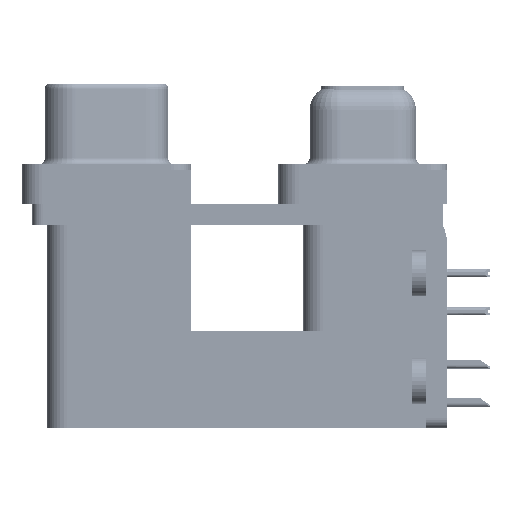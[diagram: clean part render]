
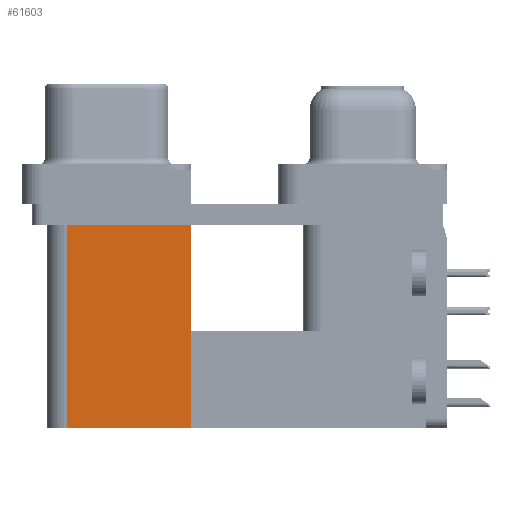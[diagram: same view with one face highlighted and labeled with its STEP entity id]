
A CAD part, left-side view. The second image highlights one B-rep face of the part: STEP entity #61603.
In plain terms, the highlighted planar face has unit normal (-1, 0, 0).
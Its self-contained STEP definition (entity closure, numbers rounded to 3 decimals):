
#1164 = VECTOR ( 'NONE', #51424, 1000. ) ;
#2717 = PLANE ( 'NONE',  #69820 ) ;
#3082 = CARTESIAN_POINT ( 'NONE',  ( 3.79, 12.775, -19.2 ) ) ;
#3786 = DIRECTION ( 'NONE',  ( 0., 1., 0. ) ) ;
#4133 = CARTESIAN_POINT ( 'NONE',  ( 3.79, 21.975, -19.2 ) ) ;
#6581 = ORIENTED_EDGE ( 'NONE', *, *, #23074, .F. ) ;
#8945 = CARTESIAN_POINT ( 'NONE',  ( 3.79, 12.775, -19.2 ) ) ;
#14215 = VECTOR ( 'NONE', #20012, 1000. ) ;
#14509 = LINE ( 'NONE', #68146, #1164 ) ;
#15348 = VECTOR ( 'NONE', #67565, 1000. ) ;
#16360 = LINE ( 'NONE', #58708, #54872 ) ;
#20012 = DIRECTION ( 'NONE',  ( 0., 0., 1. ) ) ;
#23074 = EDGE_CURVE ( 'NONE', #63557, #67993, #16360, .T. ) ;
#24173 = LINE ( 'NONE', #45863, #15348 ) ;
#28647 = EDGE_CURVE ( 'NONE', #67993, #34983, #48422, .T. ) ;
#30725 = FACE_OUTER_BOUND ( 'NONE', #31546, .T. ) ;
#31546 = EDGE_LOOP ( 'NONE', ( #35360, #55330, #6581, #67110 ) ) ;
#33035 = DIRECTION ( 'NONE',  ( 0., 1., 0. ) ) ;
#34983 = VERTEX_POINT ( 'NONE', #65165 ) ;
#35360 = ORIENTED_EDGE ( 'NONE', *, *, #40264, .T. ) ;
#40035 = VERTEX_POINT ( 'NONE', #55158 ) ;
#40264 = EDGE_CURVE ( 'NONE', #40035, #34983, #24173, .T. ) ;
#45863 = CARTESIAN_POINT ( 'NONE',  ( 3.79, 12.775, -2.5 ) ) ;
#47721 = CARTESIAN_POINT ( 'NONE',  ( 3.79, 21.975, -19.2 ) ) ;
#47839 = EDGE_CURVE ( 'NONE', #63557, #40035, #14509, .T. ) ;
#48422 = LINE ( 'NONE', #47721, #14215 ) ;
#51424 = DIRECTION ( 'NONE',  ( 0., 0., 1. ) ) ;
#54872 = VECTOR ( 'NONE', #33035, 1000. ) ;
#55158 = CARTESIAN_POINT ( 'NONE',  ( 3.79, 12.775, -2.5 ) ) ;
#55330 = ORIENTED_EDGE ( 'NONE', *, *, #28647, .F. ) ;
#56351 = DIRECTION ( 'NONE',  ( 1., 0., 0. ) ) ;
#58708 = CARTESIAN_POINT ( 'NONE',  ( 3.79, 12.775, -19.2 ) ) ;
#61603 = ADVANCED_FACE ( 'NONE', ( #30725 ), #2717, .F. ) ;
#63557 = VERTEX_POINT ( 'NONE', #8945 ) ;
#65165 = CARTESIAN_POINT ( 'NONE',  ( 3.79, 21.975, -2.5 ) ) ;
#67110 = ORIENTED_EDGE ( 'NONE', *, *, #47839, .T. ) ;
#67565 = DIRECTION ( 'NONE',  ( 0., 1., 0. ) ) ;
#67993 = VERTEX_POINT ( 'NONE', #4133 ) ;
#68146 = CARTESIAN_POINT ( 'NONE',  ( 3.79, 12.775, -19.2 ) ) ;
#69820 = AXIS2_PLACEMENT_3D ( 'NONE', #3082, #56351, #3786 ) ;
